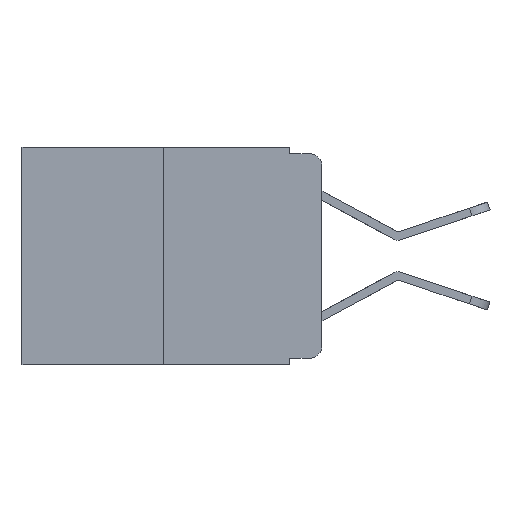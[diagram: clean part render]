
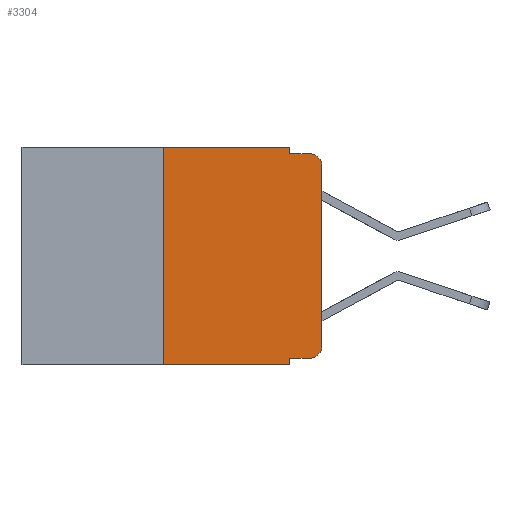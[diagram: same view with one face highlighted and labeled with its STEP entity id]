
A CAD part, left-side view. The second image highlights one B-rep face of the part: STEP entity #3304.
In plain terms, the highlighted planar face has unit normal (-1, 0, 0).
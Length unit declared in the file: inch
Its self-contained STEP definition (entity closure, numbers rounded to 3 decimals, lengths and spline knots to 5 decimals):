
#145 = ORIENTED_EDGE ( 'NONE', *, *, #190, .T. ) ;
#190 = EDGE_CURVE ( 'NONE', #6248, #11399, #10120, .T. ) ;
#687 = LINE ( 'NONE', #5369, #5618 ) ;
#1112 = EDGE_CURVE ( 'NONE', #3050, #4928, #5530, .T. ) ;
#1150 = ORIENTED_EDGE ( 'NONE', *, *, #1769, .T. ) ;
#1178 = VECTOR ( 'NONE', #8236, 39.37008 ) ;
#1289 = ORIENTED_EDGE ( 'NONE', *, *, #5554, .F. ) ;
#1577 = ORIENTED_EDGE ( 'NONE', *, *, #4728, .F. ) ;
#1659 = CIRCLE ( 'NONE', #4454, 0.02 ) ;
#1769 = EDGE_CURVE ( 'NONE', #6676, #11782, #3119, .T. ) ;
#2140 = DIRECTION ( 'NONE',  ( 0., 0., 1. ) ) ;
#2206 = LINE ( 'NONE', #11653, #11320 ) ;
#2259 = CARTESIAN_POINT ( 'NONE',  ( 0., 0.25, 0. ) ) ;
#2286 = VERTEX_POINT ( 'NONE', #10201 ) ;
#2303 = EDGE_CURVE ( 'NONE', #3613, #2286, #2206, .T. ) ;
#2629 = FACE_OUTER_BOUND ( 'NONE', #4977, .T. ) ;
#2631 = CARTESIAN_POINT ( 'NONE',  ( 0., 0., 0. ) ) ;
#2699 = DIRECTION ( 'NONE',  ( 1., 0., 0. ) ) ;
#2817 = ORIENTED_EDGE ( 'NONE', *, *, #4051, .T. ) ;
#2978 = CARTESIAN_POINT ( 'NONE',  ( 0., 0.051, -0.343 ) ) ;
#3050 = VERTEX_POINT ( 'NONE', #3365 ) ;
#3119 = LINE ( 'NONE', #7822, #4956 ) ;
#3304 = ADVANCED_FACE ( 'NONE', ( #2629 ), #8083, .F. ) ;
#3365 = CARTESIAN_POINT ( 'NONE',  ( 0., 0.25, 0. ) ) ;
#3562 = DIRECTION ( 'NONE',  ( 0., 0., -1. ) ) ;
#3599 = DIRECTION ( 'NONE',  ( -1., 0., 0. ) ) ;
#3613 = VERTEX_POINT ( 'NONE', #5194 ) ;
#3614 = CARTESIAN_POINT ( 'NONE',  ( 0., 0., -0.03 ) ) ;
#3638 = VERTEX_POINT ( 'NONE', #3614 ) ;
#4051 = EDGE_CURVE ( 'NONE', #11399, #3638, #9222, .T. ) ;
#4119 = ORIENTED_EDGE ( 'NONE', *, *, #7662, .T. ) ;
#4356 = ORIENTED_EDGE ( 'NONE', *, *, #11550, .F. ) ;
#4454 = AXIS2_PLACEMENT_3D ( 'NONE', #4747, #11095, #5679 ) ;
#4728 = EDGE_CURVE ( 'NONE', #10273, #11782, #6342, .T. ) ;
#4747 = CARTESIAN_POINT ( 'NONE',  ( 0., 0.02, -0.03 ) ) ;
#4900 = CARTESIAN_POINT ( 'NONE',  ( 0., 0.473, 0. ) ) ;
#4928 = VERTEX_POINT ( 'NONE', #8278 ) ;
#4956 = VECTOR ( 'NONE', #5200, 39.37008 ) ;
#4977 = EDGE_LOOP ( 'NONE', ( #2817, #4119, #5937, #4356, #7553, #1289, #1150, #1577, #8437, #145 ) ) ;
#5194 = CARTESIAN_POINT ( 'NONE',  ( 0., 0.051, -0.01 ) ) ;
#5200 = DIRECTION ( 'NONE',  ( 0., -1., 0. ) ) ;
#5369 = CARTESIAN_POINT ( 'NONE',  ( 0., 0.051, 0. ) ) ;
#5530 = LINE ( 'NONE', #4900, #8291 ) ;
#5554 = EDGE_CURVE ( 'NONE', #6676, #3050, #11380, .T. ) ;
#5618 = VECTOR ( 'NONE', #3562, 39.37008 ) ;
#5679 = DIRECTION ( 'NONE',  ( 0., 0., -1. ) ) ;
#5773 = CARTESIAN_POINT ( 'NONE',  ( 0., 0.02, -0.313 ) ) ;
#5820 = LINE ( 'NONE', #11734, #1178 ) ;
#5937 = ORIENTED_EDGE ( 'NONE', *, *, #2303, .F. ) ;
#6248 = VERTEX_POINT ( 'NONE', #6334 ) ;
#6334 = CARTESIAN_POINT ( 'NONE',  ( 0., 0.02, -0.333 ) ) ;
#6342 = LINE ( 'NONE', #8192, #6639 ) ;
#6415 = CARTESIAN_POINT ( 'NONE',  ( 0., 0., -0.313 ) ) ;
#6571 = DIRECTION ( 'NONE',  ( 0., -1., 0. ) ) ;
#6639 = VECTOR ( 'NONE', #10141, 39.37008 ) ;
#6676 = VERTEX_POINT ( 'NONE', #10572 ) ;
#7016 = AXIS2_PLACEMENT_3D ( 'NONE', #5773, #3599, #9500 ) ;
#7553 = ORIENTED_EDGE ( 'NONE', *, *, #1112, .F. ) ;
#7662 = EDGE_CURVE ( 'NONE', #3638, #2286, #1659, .T. ) ;
#7822 = CARTESIAN_POINT ( 'NONE',  ( 0., 0.473, -0.343 ) ) ;
#8054 = DIRECTION ( 'NONE',  ( 0., 0., 1. ) ) ;
#8083 = PLANE ( 'NONE',  #10852 ) ;
#8101 = CARTESIAN_POINT ( 'NONE',  ( 0., 0.473, 0. ) ) ;
#8192 = CARTESIAN_POINT ( 'NONE',  ( 0., 0.051, 0. ) ) ;
#8236 = DIRECTION ( 'NONE',  ( 0., -1., 0. ) ) ;
#8259 = CARTESIAN_POINT ( 'NONE',  ( 0., 0.051, -0.333 ) ) ;
#8278 = CARTESIAN_POINT ( 'NONE',  ( 0., 0.051, 0. ) ) ;
#8291 = VECTOR ( 'NONE', #6571, 39.37008 ) ;
#8437 = ORIENTED_EDGE ( 'NONE', *, *, #9634, .T. ) ;
#9037 = VECTOR ( 'NONE', #2140, 39.37008 ) ;
#9222 = LINE ( 'NONE', #2631, #10999 ) ;
#9500 = DIRECTION ( 'NONE',  ( 0., 0., -1. ) ) ;
#9634 = EDGE_CURVE ( 'NONE', #10273, #6248, #5820, .T. ) ;
#9650 = DIRECTION ( 'NONE',  ( 0., 0., -1. ) ) ;
#10120 = CIRCLE ( 'NONE', #7016, 0.02 ) ;
#10141 = DIRECTION ( 'NONE',  ( 0., 0., -1. ) ) ;
#10201 = CARTESIAN_POINT ( 'NONE',  ( 0., 0.02, -0.01 ) ) ;
#10273 = VERTEX_POINT ( 'NONE', #8259 ) ;
#10572 = CARTESIAN_POINT ( 'NONE',  ( 0., 0.25, -0.343 ) ) ;
#10852 = AXIS2_PLACEMENT_3D ( 'NONE', #8101, #2699, #9650 ) ;
#10999 = VECTOR ( 'NONE', #8054, 39.37008 ) ;
#11095 = DIRECTION ( 'NONE',  ( -1., 0., 0. ) ) ;
#11320 = VECTOR ( 'NONE', #11639, 39.37008 ) ;
#11380 = LINE ( 'NONE', #2259, #9037 ) ;
#11399 = VERTEX_POINT ( 'NONE', #6415 ) ;
#11550 = EDGE_CURVE ( 'NONE', #4928, #3613, #687, .T. ) ;
#11639 = DIRECTION ( 'NONE',  ( 0., -1., 0. ) ) ;
#11653 = CARTESIAN_POINT ( 'NONE',  ( 0., 0.051, -0.01 ) ) ;
#11734 = CARTESIAN_POINT ( 'NONE',  ( 0., 0.051, -0.333 ) ) ;
#11782 = VERTEX_POINT ( 'NONE', #2978 ) ;
